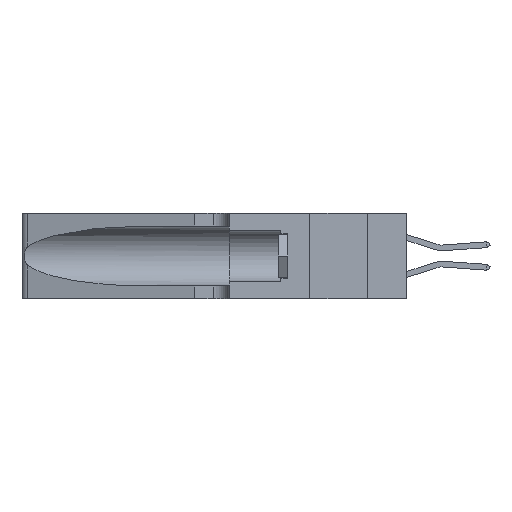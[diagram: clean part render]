
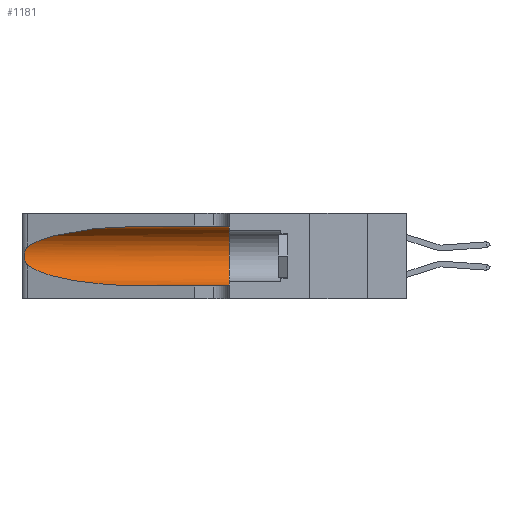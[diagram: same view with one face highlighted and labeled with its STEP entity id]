
A CAD part, left-side view. The second image highlights one B-rep face of the part: STEP entity #1181.
In plain terms, the highlighted cylindrical face has radius 3.308 mm (diameter 6.617 mm), a partial arc.
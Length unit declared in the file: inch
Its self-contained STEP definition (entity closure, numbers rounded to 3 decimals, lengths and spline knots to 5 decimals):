
#474 = DIRECTION ( 'NONE',  ( 0., -1., 0. ) ) ;
#928 = CARTESIAN_POINT ( 'NONE',  ( 0.25487, 1.22718, 0.22369 ) ) ;
#1181 = ADVANCED_FACE ( 'NONE', ( #16869 ), #2594, .F. ) ;
#1250 = DIRECTION ( 'NONE',  ( 0., -1., 0. ) ) ;
#1267 = CARTESIAN_POINT ( 'NONE',  ( 0.1305, 0.35, 0.185 ) ) ;
#1778 = EDGE_CURVE ( 'NONE', #3092, #21305, #17236, .T. ) ;
#2594 = CYLINDRICAL_SURFACE ( 'NONE', #30925, 0.13025 ) ;
#2644 =( BOUNDED_CURVE ( )  B_SPLINE_CURVE ( 3, ( #24547, #14665, #13940, #8497 ),
 .UNSPECIFIED., .F., .F. ) 
 B_SPLINE_CURVE_WITH_KNOTS ( ( 4, 4 ),
 ( 3.44316, 4.71239 ),
 .UNSPECIFIED. ) 
 CURVE ( )  GEOMETRIC_REPRESENTATION_ITEM ( )  RATIONAL_B_SPLINE_CURVE ( ( 1., 0.87, 0.87, 1. ) ) 
 REPRESENTATION_ITEM ( '' )  );
#3092 = VERTEX_POINT ( 'NONE', #5184 ) ;
#4451 = LINE ( 'NONE', #29342, #15179 ) ;
#4452 = CARTESIAN_POINT ( 'NONE',  ( 0.25854, 1.2359, 0.20912 ) ) ;
#4720 = CARTESIAN_POINT ( 'NONE',  ( 0.25487, 1.22718, 0.14631 ) ) ;
#5184 = CARTESIAN_POINT ( 'NONE',  ( 0.1305, 0.72297, 0.31525 ) ) ;
#5276 = CARTESIAN_POINT ( 'NONE',  ( 0.25789, 1.23486, 0.15765 ) ) ;
#6475 = CARTESIAN_POINT ( 'NONE',  ( 0.25487, 1.22718, 0.22369 ) ) ;
#8497 = CARTESIAN_POINT ( 'NONE',  ( 0.1305, 0.72297, 0.05475 ) ) ;
#8757 = CARTESIAN_POINT ( 'NONE',  ( 0.1305, 0.72297, 0.05475 ) ) ;
#9139 =( BOUNDED_CURVE ( )  B_SPLINE_CURVE ( 3, ( #32555, #30199, #29574, #6475 ),
 .UNSPECIFIED., .F., .T. ) 
 B_SPLINE_CURVE_WITH_KNOTS ( ( 4, 4 ),
 ( 1.5708, 2.84003 ),
 .UNSPECIFIED. ) 
 CURVE ( )  GEOMETRIC_REPRESENTATION_ITEM ( )  RATIONAL_B_SPLINE_CURVE ( ( 1., 0.87, 0.87, 1. ) ) 
 REPRESENTATION_ITEM ( '' )  );
#10957 = VERTEX_POINT ( 'NONE', #4720 ) ;
#12122 = VERTEX_POINT ( 'NONE', #928 ) ;
#12371 = CIRCLE ( 'NONE', #30668, 0.13025 ) ;
#12464 = ORIENTED_EDGE ( 'NONE', *, *, #16657, .T. ) ;
#13940 = CARTESIAN_POINT ( 'NONE',  ( 0.18966, 0.96281, 0.05475 ) ) ;
#13941 = ORIENTED_EDGE ( 'NONE', *, *, #17721, .T. ) ;
#14665 = CARTESIAN_POINT ( 'NONE',  ( 0.2373, 1.15595, 0.08982 ) ) ;
#15095 = CARTESIAN_POINT ( 'NONE',  ( 0.26075, 1.23896, 0.178 ) ) ;
#15179 = VECTOR ( 'NONE', #1250, 39.37008 ) ;
#15397 = ORIENTED_EDGE ( 'NONE', *, *, #31973, .T. ) ;
#15718 = CARTESIAN_POINT ( 'NONE',  ( 0.1305, 1.61858, 0.185 ) ) ;
#16475 = DIRECTION ( 'NONE',  ( 0., 0., 1. ) ) ;
#16657 = EDGE_CURVE ( 'NONE', #3092, #12122, #9139, .T. ) ;
#16735 = CARTESIAN_POINT ( 'NONE',  ( 0.1305, 0.35, 0.31525 ) ) ;
#16869 = FACE_OUTER_BOUND ( 'NONE', #20816, .T. ) ;
#17236 = LINE ( 'NONE', #28154, #27821 ) ;
#17414 = CARTESIAN_POINT ( 'NONE',  ( 0.25787, 1.23484, 0.2124 ) ) ;
#17721 = EDGE_CURVE ( 'NONE', #12122, #10957, #27153, .T. ) ;
#17950 = ORIENTED_EDGE ( 'NONE', *, *, #24441, .F. ) ;
#20240 = VERTEX_POINT ( 'NONE', #25220 ) ;
#20459 = CARTESIAN_POINT ( 'NONE',  ( 0.26017, 1.23833, 0.17102 ) ) ;
#20816 = EDGE_LOOP ( 'NONE', ( #12464, #13941, #29626, #15397, #17950, #32352 ) ) ;
#21305 = VERTEX_POINT ( 'NONE', #16735 ) ;
#21652 = DIRECTION ( 'NONE',  ( 0., 1., 0. ) ) ;
#21780 = EDGE_CURVE ( 'NONE', #10957, #26967, #2644, .T. ) ;
#23067 = DIRECTION ( 'NONE',  ( 0., 0., -1. ) ) ;
#24441 = EDGE_CURVE ( 'NONE', #21305, #20240, #12371, .T. ) ;
#24547 = CARTESIAN_POINT ( 'NONE',  ( 0.25487, 1.22718, 0.14631 ) ) ;
#25220 = CARTESIAN_POINT ( 'NONE',  ( 0.1305, 0.35, 0.05475 ) ) ;
#26967 = VERTEX_POINT ( 'NONE', #8757 ) ;
#27153 = B_SPLINE_CURVE_WITH_KNOTS ( 'NONE', 3,
 ( #29388, #32069, #27406, #17414, #4452, #30064, #27187, #15095, #20459, #30368, #5276, #28027, #30579, #30992 ),
 .UNSPECIFIED., .F., .F.,
 ( 4, 2, 2, 2, 2, 2, 4 ),
 ( 0., 0.00027, 0.00053, 0.00107, 0.0016, 0.00187, 0.00214 ),
 .UNSPECIFIED. ) ;
#27187 = CARTESIAN_POINT ( 'NONE',  ( 0.26075, 1.23896, 0.19203 ) ) ;
#27406 = CARTESIAN_POINT ( 'NONE',  ( 0.25639, 1.23184, 0.21858 ) ) ;
#27821 = VECTOR ( 'NONE', #30497, 39.37008 ) ;
#28027 = CARTESIAN_POINT ( 'NONE',  ( 0.25639, 1.23186, 0.15144 ) ) ;
#28154 = CARTESIAN_POINT ( 'NONE',  ( 0.1305, 1.61858, 0.31525 ) ) ;
#29342 = CARTESIAN_POINT ( 'NONE',  ( 0.1305, 1.61858, 0.05475 ) ) ;
#29388 = CARTESIAN_POINT ( 'NONE',  ( 0.25487, 1.22718, 0.22369 ) ) ;
#29574 = CARTESIAN_POINT ( 'NONE',  ( 0.2373, 1.15595, 0.28018 ) ) ;
#29626 = ORIENTED_EDGE ( 'NONE', *, *, #21780, .T. ) ;
#30064 = CARTESIAN_POINT ( 'NONE',  ( 0.26018, 1.23835, 0.19895 ) ) ;
#30199 = CARTESIAN_POINT ( 'NONE',  ( 0.18966, 0.96281, 0.31525 ) ) ;
#30368 = CARTESIAN_POINT ( 'NONE',  ( 0.25856, 1.23593, 0.16098 ) ) ;
#30497 = DIRECTION ( 'NONE',  ( 0., -1., 0. ) ) ;
#30579 = CARTESIAN_POINT ( 'NONE',  ( 0.25555, 1.22993, 0.14849 ) ) ;
#30668 = AXIS2_PLACEMENT_3D ( 'NONE', #1267, #21652, #16475 ) ;
#30925 = AXIS2_PLACEMENT_3D ( 'NONE', #15718, #474, #23067 ) ;
#30992 = CARTESIAN_POINT ( 'NONE',  ( 0.25487, 1.22718, 0.14631 ) ) ;
#31973 = EDGE_CURVE ( 'NONE', #26967, #20240, #4451, .T. ) ;
#32069 = CARTESIAN_POINT ( 'NONE',  ( 0.25555, 1.22994, 0.2215 ) ) ;
#32352 = ORIENTED_EDGE ( 'NONE', *, *, #1778, .F. ) ;
#32555 = CARTESIAN_POINT ( 'NONE',  ( 0.1305, 0.72297, 0.31525 ) ) ;
